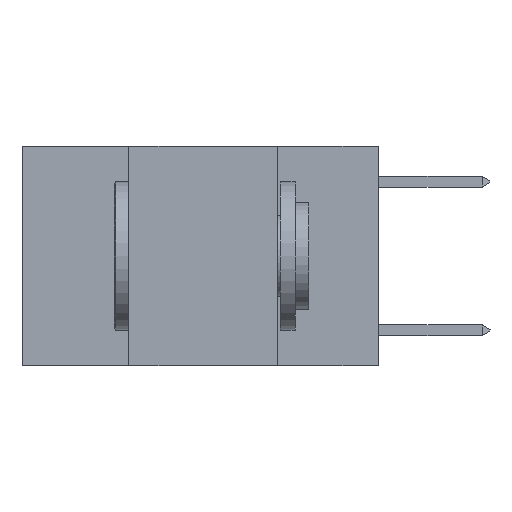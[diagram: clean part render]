
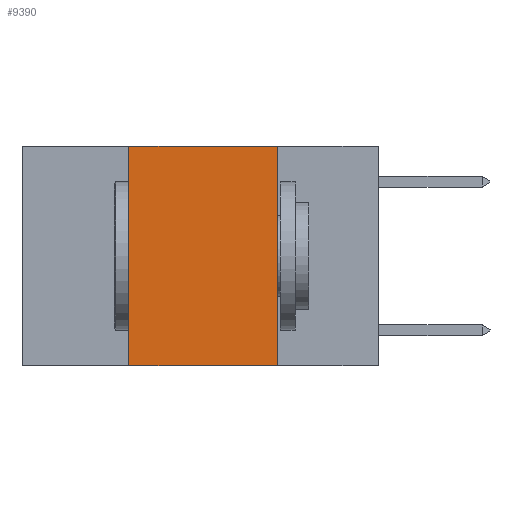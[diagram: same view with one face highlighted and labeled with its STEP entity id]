
A CAD part, left-side view. The second image highlights one B-rep face of the part: STEP entity #9390.
In plain terms, the highlighted planar face has unit normal (-1, 0, 0).
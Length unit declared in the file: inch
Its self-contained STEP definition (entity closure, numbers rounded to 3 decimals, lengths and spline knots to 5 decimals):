
#313 = VERTEX_POINT ( 'NONE', #16441 ) ;
#473 = ORIENTED_EDGE ( 'NONE', *, *, #20908, .F. ) ;
#1226 = DIRECTION ( 'NONE',  ( 0., 0., -1. ) ) ;
#1330 = DIRECTION ( 'NONE',  ( 0., 0., -1. ) ) ;
#1783 = AXIS2_PLACEMENT_3D ( 'NONE', #22760, #12442, #1330 ) ;
#2713 = CARTESIAN_POINT ( 'NONE',  ( 0., 0.17, 0. ) ) ;
#6979 = CARTESIAN_POINT ( 'NONE',  ( 0., 0.17, 0. ) ) ;
#7574 = CARTESIAN_POINT ( 'NONE',  ( 0., 0.42, 0. ) ) ;
#8236 = DIRECTION ( 'NONE',  ( 0., -1., 0. ) ) ;
#8552 = VERTEX_POINT ( 'NONE', #2713 ) ;
#8934 = LINE ( 'NONE', #7574, #21893 ) ;
#9390 = ADVANCED_FACE ( 'NONE', ( #23031 ), #21105, .F. ) ;
#9399 = DIRECTION ( 'NONE',  ( 0., 0., 1. ) ) ;
#9878 = VERTEX_POINT ( 'NONE', #11865 ) ;
#10524 = ORIENTED_EDGE ( 'NONE', *, *, #21984, .F. ) ;
#11370 = CARTESIAN_POINT ( 'NONE',  ( 0., 0.6, -0.37 ) ) ;
#11865 = CARTESIAN_POINT ( 'NONE',  ( 0., 0.42, 0. ) ) ;
#11887 = CARTESIAN_POINT ( 'NONE',  ( 0., 0.6, 0. ) ) ;
#12303 = VECTOR ( 'NONE', #1226, 39.37008 ) ;
#12442 = DIRECTION ( 'NONE',  ( 1., 0., 0. ) ) ;
#12495 = LINE ( 'NONE', #11887, #21255 ) ;
#13158 = CARTESIAN_POINT ( 'NONE',  ( 0., 0.17, -0.37 ) ) ;
#14304 = ORIENTED_EDGE ( 'NONE', *, *, #19792, .T. ) ;
#16441 = CARTESIAN_POINT ( 'NONE',  ( 0., 0.42, -0.37 ) ) ;
#16816 = DIRECTION ( 'NONE',  ( 0., -1., 0. ) ) ;
#16823 = VERTEX_POINT ( 'NONE', #13158 ) ;
#17217 = LINE ( 'NONE', #11370, #21714 ) ;
#18757 = EDGE_LOOP ( 'NONE', ( #10524, #21908, #473, #14304 ) ) ;
#18976 = EDGE_CURVE ( 'NONE', #9878, #8552, #12495, .T. ) ;
#19792 = EDGE_CURVE ( 'NONE', #313, #16823, #17217, .T. ) ;
#20908 = EDGE_CURVE ( 'NONE', #313, #9878, #8934, .T. ) ;
#21096 = LINE ( 'NONE', #6979, #12303 ) ;
#21105 = PLANE ( 'NONE',  #1783 ) ;
#21255 = VECTOR ( 'NONE', #8236, 39.37008 ) ;
#21714 = VECTOR ( 'NONE', #16816, 39.37008 ) ;
#21893 = VECTOR ( 'NONE', #9399, 39.37008 ) ;
#21908 = ORIENTED_EDGE ( 'NONE', *, *, #18976, .F. ) ;
#21984 = EDGE_CURVE ( 'NONE', #8552, #16823, #21096, .T. ) ;
#22760 = CARTESIAN_POINT ( 'NONE',  ( 0., 0.6, 0. ) ) ;
#23031 = FACE_OUTER_BOUND ( 'NONE', #18757, .T. ) ;
